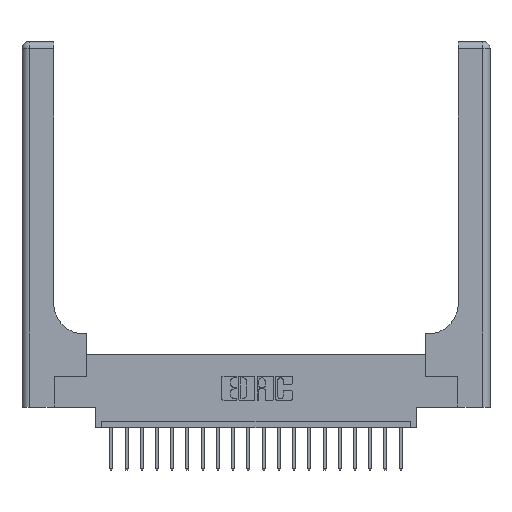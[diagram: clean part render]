
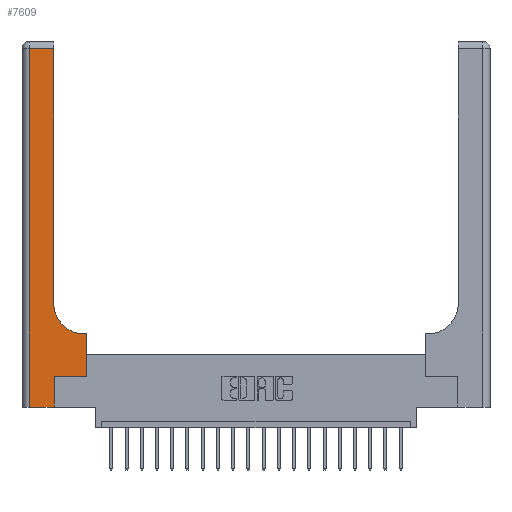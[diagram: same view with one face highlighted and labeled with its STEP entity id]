
A CAD part, top view. The second image highlights one B-rep face of the part: STEP entity #7609.
In plain terms, the highlighted planar face has unit normal (0, 0, 1).
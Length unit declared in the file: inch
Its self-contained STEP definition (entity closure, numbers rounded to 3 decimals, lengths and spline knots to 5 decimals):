
#632 = CARTESIAN_POINT ( 'NONE',  ( 0.06, 2.94, 0.37 ) ) ;
#889 = EDGE_CURVE ( 'NONE', #20611, #5411, #15833, .T. ) ;
#1020 = ORIENTED_EDGE ( 'NONE', *, *, #6537, .T. ) ;
#1137 = LINE ( 'NONE', #11802, #10655 ) ;
#1587 = DIRECTION ( 'NONE',  ( 0., 0., -1. ) ) ;
#1609 = CARTESIAN_POINT ( 'NONE',  ( 0.51, 0.6, 0.37 ) ) ;
#2742 = ORIENTED_EDGE ( 'NONE', *, *, #7852, .T. ) ;
#2934 = DIRECTION ( 'NONE',  ( -1., 0., 0. ) ) ;
#3676 = DIRECTION ( 'NONE',  ( 1., 0., 0. ) ) ;
#3855 = CARTESIAN_POINT ( 'NONE',  ( 0.528, 0.6, 0.37 ) ) ;
#4271 = ORIENTED_EDGE ( 'NONE', *, *, #7758, .T. ) ;
#4374 = CARTESIAN_POINT ( 'NONE',  ( 0., 0., 0.37 ) ) ;
#4478 = DIRECTION ( 'NONE',  ( -1., 0., 0. ) ) ;
#4984 = LINE ( 'NONE', #16108, #20002 ) ;
#5222 = EDGE_CURVE ( 'NONE', #18145, #18022, #8650, .T. ) ;
#5411 = VERTEX_POINT ( 'NONE', #9273 ) ;
#5533 = VERTEX_POINT ( 'NONE', #3855 ) ;
#5732 = VERTEX_POINT ( 'NONE', #19546 ) ;
#6350 = CARTESIAN_POINT ( 'NONE',  ( 0., 3., 0.37 ) ) ;
#6537 = EDGE_CURVE ( 'NONE', #16515, #10289, #18309, .T. ) ;
#6712 = DIRECTION ( 'NONE',  ( -1., 0., 0. ) ) ;
#6987 = FACE_OUTER_BOUND ( 'NONE', #16162, .T. ) ;
#7256 = CARTESIAN_POINT ( 'NONE',  ( 0.06, 0., 0.37 ) ) ;
#7475 = CARTESIAN_POINT ( 'NONE',  ( 0.265, 0., 0.37 ) ) ;
#7599 = ORIENTED_EDGE ( 'NONE', *, *, #5222, .T. ) ;
#7609 = ADVANCED_FACE ( 'NONE', ( #6987 ), #10919, .F. ) ;
#7758 = EDGE_CURVE ( 'NONE', #5732, #13024, #4984, .T. ) ;
#7852 = EDGE_CURVE ( 'NONE', #5533, #18145, #14740, .T. ) ;
#8613 = ORIENTED_EDGE ( 'NONE', *, *, #8845, .T. ) ;
#8650 = CIRCLE ( 'NONE', #20390, 0.25 ) ;
#8845 = EDGE_CURVE ( 'NONE', #10289, #20611, #13184, .T. ) ;
#9057 = CARTESIAN_POINT ( 'NONE',  ( 0.26, 0.6, 0.37 ) ) ;
#9132 = CARTESIAN_POINT ( 'NONE',  ( 0.265, 0.25, 0.37 ) ) ;
#9273 = CARTESIAN_POINT ( 'NONE',  ( 0.528, 0.25, 0.37 ) ) ;
#9733 = CARTESIAN_POINT ( 'NONE',  ( 0.06, 3., 0.37 ) ) ;
#9771 = CARTESIAN_POINT ( 'NONE',  ( 0.51, 0.85, 0.37 ) ) ;
#10042 = EDGE_CURVE ( 'NONE', #13024, #16515, #12105, .T. ) ;
#10289 = VERTEX_POINT ( 'NONE', #7475 ) ;
#10390 = VECTOR ( 'NONE', #12705, 39.37008 ) ;
#10655 = VECTOR ( 'NONE', #18264, 39.37008 ) ;
#10919 = PLANE ( 'NONE',  #17258 ) ;
#10951 = EDGE_CURVE ( 'NONE', #18022, #5732, #20096, .T. ) ;
#10979 = VECTOR ( 'NONE', #2934, 39.37008 ) ;
#11378 = DIRECTION ( 'NONE',  ( 1., 0., 0. ) ) ;
#11744 = ORIENTED_EDGE ( 'NONE', *, *, #10951, .T. ) ;
#11790 = VECTOR ( 'NONE', #3676, 39.37008 ) ;
#11802 = CARTESIAN_POINT ( 'NONE',  ( 0.528, 0.25, 0.37 ) ) ;
#12105 = LINE ( 'NONE', #9733, #10390 ) ;
#12373 = CARTESIAN_POINT ( 'NONE',  ( 0.265, 0., 0.37 ) ) ;
#12500 = CARTESIAN_POINT ( 'NONE',  ( 0.26, 3., 0.37 ) ) ;
#12564 = DIRECTION ( 'NONE',  ( 0., 0., -1. ) ) ;
#12699 = ORIENTED_EDGE ( 'NONE', *, *, #19886, .T. ) ;
#12705 = DIRECTION ( 'NONE',  ( 0., -1., 0. ) ) ;
#13024 = VERTEX_POINT ( 'NONE', #632 ) ;
#13184 = LINE ( 'NONE', #12373, #18716 ) ;
#13449 = ORIENTED_EDGE ( 'NONE', *, *, #10042, .T. ) ;
#14185 = DIRECTION ( 'NONE',  ( 0., 1., 0. ) ) ;
#14740 = LINE ( 'NONE', #9057, #10979 ) ;
#15478 = CARTESIAN_POINT ( 'NONE',  ( 0.26, 0.85, 0.37 ) ) ;
#15798 = VECTOR ( 'NONE', #17202, 39.37008 ) ;
#15833 = LINE ( 'NONE', #9132, #11790 ) ;
#16108 = CARTESIAN_POINT ( 'NONE',  ( 0., 2.94, 0.37 ) ) ;
#16162 = EDGE_LOOP ( 'NONE', ( #11744, #4271, #13449, #1020, #8613, #17675, #12699, #2742, #7599 ) ) ;
#16515 = VERTEX_POINT ( 'NONE', #7256 ) ;
#16847 = VECTOR ( 'NONE', #14185, 39.37008 ) ;
#17202 = DIRECTION ( 'NONE',  ( 1., 0., 0. ) ) ;
#17258 = AXIS2_PLACEMENT_3D ( 'NONE', #6350, #12564, #4478 ) ;
#17675 = ORIENTED_EDGE ( 'NONE', *, *, #889, .T. ) ;
#18022 = VERTEX_POINT ( 'NONE', #15478 ) ;
#18145 = VERTEX_POINT ( 'NONE', #1609 ) ;
#18264 = DIRECTION ( 'NONE',  ( 0., 1., 0. ) ) ;
#18309 = LINE ( 'NONE', #4374, #15798 ) ;
#18716 = VECTOR ( 'NONE', #18911, 39.37008 ) ;
#18911 = DIRECTION ( 'NONE',  ( 0., 1., 0. ) ) ;
#19546 = CARTESIAN_POINT ( 'NONE',  ( 0.26, 2.94, 0.37 ) ) ;
#19886 = EDGE_CURVE ( 'NONE', #5411, #5533, #1137, .T. ) ;
#19907 = CARTESIAN_POINT ( 'NONE',  ( 0.265, 0.25, 0.37 ) ) ;
#20002 = VECTOR ( 'NONE', #6712, 39.37008 ) ;
#20096 = LINE ( 'NONE', #12500, #16847 ) ;
#20390 = AXIS2_PLACEMENT_3D ( 'NONE', #9771, #1587, #11378 ) ;
#20611 = VERTEX_POINT ( 'NONE', #19907 ) ;
